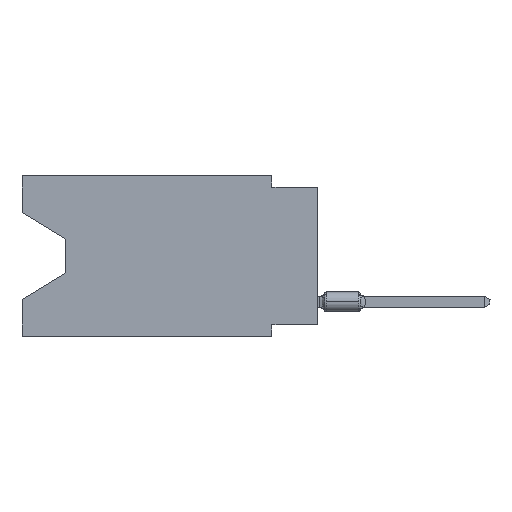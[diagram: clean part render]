
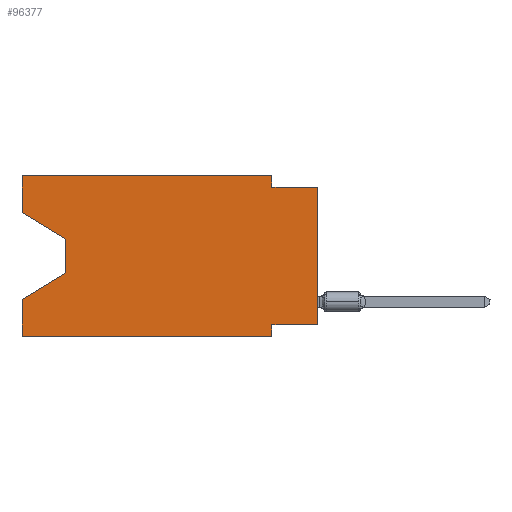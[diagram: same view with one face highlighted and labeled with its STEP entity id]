
A CAD part, left-side view. The second image highlights one B-rep face of the part: STEP entity #96377.
In plain terms, the highlighted planar face has unit normal (-1, 0, 0).
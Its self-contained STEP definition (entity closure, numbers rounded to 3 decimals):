
#4000 = EDGE_CURVE ( 'NONE', #24201, #12619, #29725, .T. ) ;
#5384 = LINE ( 'NONE', #61305, #67205 ) ;
#8667 = ORIENTED_EDGE ( 'NONE', *, *, #61540, .F. ) ;
#9030 = VERTEX_POINT ( 'NONE', #35441 ) ;
#9311 = CARTESIAN_POINT ( 'NONE',  ( 0., 2.54, 0. ) ) ;
#9453 = VECTOR ( 'NONE', #21239, 1000. ) ;
#11814 = AXIS2_PLACEMENT_3D ( 'NONE', #53244, #22499, #74934 ) ;
#12328 = CARTESIAN_POINT ( 'NONE',  ( 0., 16.383, -8.89 ) ) ;
#12422 = CARTESIAN_POINT ( 'NONE',  ( 0., 13.97, -3.505 ) ) ;
#12619 = VERTEX_POINT ( 'NONE', #95103 ) ;
#12642 = LINE ( 'NONE', #27778, #80653 ) ;
#12911 = DIRECTION ( 'NONE',  ( 0., 0., 1. ) ) ;
#13414 = CARTESIAN_POINT ( 'NONE',  ( 0., 0., 0. ) ) ;
#13535 = EDGE_CURVE ( 'NONE', #70506, #37479, #15150, .T. ) ;
#14707 = ORIENTED_EDGE ( 'NONE', *, *, #13535, .F. ) ;
#14742 = EDGE_CURVE ( 'NONE', #97646, #92942, #74917, .T. ) ;
#15150 = LINE ( 'NONE', #37864, #9453 ) ;
#18171 = VERTEX_POINT ( 'NONE', #9311 ) ;
#20701 = CARTESIAN_POINT ( 'NONE',  ( 0., 16.383, 0. ) ) ;
#20739 = DIRECTION ( 'NONE',  ( 0., -1., 0. ) ) ;
#20924 = VECTOR ( 'NONE', #30051, 1000. ) ;
#21239 = DIRECTION ( 'NONE',  ( 0., 0., -1. ) ) ;
#22499 = DIRECTION ( 'NONE',  ( 1., 0., 0. ) ) ;
#24201 = VERTEX_POINT ( 'NONE', #43690 ) ;
#24605 = CARTESIAN_POINT ( 'NONE',  ( 0., 16.383, -6.852 ) ) ;
#25156 = VERTEX_POINT ( 'NONE', #47427 ) ;
#25618 = VECTOR ( 'NONE', #96000, 1000. ) ;
#26809 = DIRECTION ( 'NONE',  ( 0., 0., -1. ) ) ;
#26849 = ORIENTED_EDGE ( 'NONE', *, *, #30157, .T. ) ;
#27102 = EDGE_CURVE ( 'NONE', #25156, #48154, #12642, .T. ) ;
#27778 = CARTESIAN_POINT ( 'NONE',  ( 0., 16.383, 0. ) ) ;
#28011 = CARTESIAN_POINT ( 'NONE',  ( 0., 13.97, -5.385 ) ) ;
#28906 = CARTESIAN_POINT ( 'NONE',  ( 0., 0., -8.255 ) ) ;
#29148 = ORIENTED_EDGE ( 'NONE', *, *, #45653, .F. ) ;
#29725 = LINE ( 'NONE', #76069, #42276 ) ;
#30051 = DIRECTION ( 'NONE',  ( 0., 0., 1. ) ) ;
#30157 = EDGE_CURVE ( 'NONE', #25156, #9030, #97678, .T. ) ;
#30634 = VECTOR ( 'NONE', #26809, 1000. ) ;
#32285 = LINE ( 'NONE', #12422, #36647 ) ;
#34878 = CARTESIAN_POINT ( 'NONE',  ( 0., 2.54, 0. ) ) ;
#35441 = CARTESIAN_POINT ( 'NONE',  ( 0., 13.97, -3.505 ) ) ;
#35876 = LINE ( 'NONE', #67103, #85628 ) ;
#36561 = ORIENTED_EDGE ( 'NONE', *, *, #84412, .T. ) ;
#36647 = VECTOR ( 'NONE', #65856, 1000. ) ;
#36966 = VECTOR ( 'NONE', #12911, 1000. ) ;
#37479 = VERTEX_POINT ( 'NONE', #87534 ) ;
#37864 = CARTESIAN_POINT ( 'NONE',  ( 0., 2.54, -8.89 ) ) ;
#39270 = DIRECTION ( 'NONE',  ( 0., -1., 0. ) ) ;
#40827 = CARTESIAN_POINT ( 'NONE',  ( 0., 2.54, -8.255 ) ) ;
#42276 = VECTOR ( 'NONE', #39270, 1000. ) ;
#43690 = CARTESIAN_POINT ( 'NONE',  ( 0., 2.54, -0.635 ) ) ;
#45653 = EDGE_CURVE ( 'NONE', #63135, #70506, #5384, .T. ) ;
#46171 = ORIENTED_EDGE ( 'NONE', *, *, #4000, .F. ) ;
#47427 = CARTESIAN_POINT ( 'NONE',  ( 0., 16.383, -2.038 ) ) ;
#48154 = VERTEX_POINT ( 'NONE', #84189 ) ;
#50703 = EDGE_CURVE ( 'NONE', #97646, #37479, #35876, .T. ) ;
#51859 = DIRECTION ( 'NONE',  ( 0., -0.855, -0.519 ) ) ;
#53244 = CARTESIAN_POINT ( 'NONE',  ( 0., 16.383, 0. ) ) ;
#53739 = FACE_OUTER_BOUND ( 'NONE', #76196, .T. ) ;
#57558 = ORIENTED_EDGE ( 'NONE', *, *, #90382, .T. ) ;
#59411 = CARTESIAN_POINT ( 'NONE',  ( 0., 16.383, -2.038 ) ) ;
#59505 = DIRECTION ( 'NONE',  ( 0., -1., 0. ) ) ;
#59524 = DIRECTION ( 'NONE',  ( 0., 0., 1. ) ) ;
#60547 = EDGE_CURVE ( 'NONE', #85233, #92942, #97007, .T. ) ;
#61305 = CARTESIAN_POINT ( 'NONE',  ( 0., 0., -8.255 ) ) ;
#61540 = EDGE_CURVE ( 'NONE', #48154, #18171, #89731, .T. ) ;
#61944 = ORIENTED_EDGE ( 'NONE', *, *, #91007, .F. ) ;
#63135 = VERTEX_POINT ( 'NONE', #28906 ) ;
#65856 = DIRECTION ( 'NONE',  ( 0., 0., -1. ) ) ;
#67103 = CARTESIAN_POINT ( 'NONE',  ( 0., 16.383, -8.89 ) ) ;
#67205 = VECTOR ( 'NONE', #76428, 1000. ) ;
#70506 = VERTEX_POINT ( 'NONE', #40827 ) ;
#73911 = CARTESIAN_POINT ( 'NONE',  ( 0., 16.383, 0. ) ) ;
#74917 = LINE ( 'NONE', #73911, #36966 ) ;
#74934 = DIRECTION ( 'NONE',  ( 0., 0., -1. ) ) ;
#76069 = CARTESIAN_POINT ( 'NONE',  ( 0., 0., -0.635 ) ) ;
#76196 = EDGE_LOOP ( 'NONE', ( #26849, #36561, #86576, #77764, #98702, #14707, #29148, #57558, #46171, #61944, #8667, #98672 ) ) ;
#76428 = DIRECTION ( 'NONE',  ( 0., 1., 0. ) ) ;
#77764 = ORIENTED_EDGE ( 'NONE', *, *, #14742, .F. ) ;
#79929 = VECTOR ( 'NONE', #51859, 1000. ) ;
#80653 = VECTOR ( 'NONE', #59524, 1000. ) ;
#82483 = PLANE ( 'NONE',  #11814 ) ;
#84189 = CARTESIAN_POINT ( 'NONE',  ( 0., 16.383, 0. ) ) ;
#84412 = EDGE_CURVE ( 'NONE', #9030, #85233, #32285, .T. ) ;
#85233 = VERTEX_POINT ( 'NONE', #96333 ) ;
#85628 = VECTOR ( 'NONE', #20739, 1000. ) ;
#86576 = ORIENTED_EDGE ( 'NONE', *, *, #60547, .T. ) ;
#87534 = CARTESIAN_POINT ( 'NONE',  ( 0., 2.54, -8.89 ) ) ;
#89731 = LINE ( 'NONE', #20701, #91658 ) ;
#90382 = EDGE_CURVE ( 'NONE', #63135, #12619, #99055, .T. ) ;
#91007 = EDGE_CURVE ( 'NONE', #18171, #24201, #95812, .T. ) ;
#91658 = VECTOR ( 'NONE', #59505, 1000. ) ;
#92942 = VERTEX_POINT ( 'NONE', #24605 ) ;
#95103 = CARTESIAN_POINT ( 'NONE',  ( 0., 0., -0.635 ) ) ;
#95812 = LINE ( 'NONE', #34878, #30634 ) ;
#96000 = DIRECTION ( 'NONE',  ( 0., 0.855, -0.519 ) ) ;
#96333 = CARTESIAN_POINT ( 'NONE',  ( 0., 13.97, -5.385 ) ) ;
#96377 = ADVANCED_FACE ( 'NONE', ( #53739 ), #82483, .F. ) ;
#97007 = LINE ( 'NONE', #28011, #25618 ) ;
#97646 = VERTEX_POINT ( 'NONE', #12328 ) ;
#97678 = LINE ( 'NONE', #59411, #79929 ) ;
#98672 = ORIENTED_EDGE ( 'NONE', *, *, #27102, .F. ) ;
#98702 = ORIENTED_EDGE ( 'NONE', *, *, #50703, .T. ) ;
#99055 = LINE ( 'NONE', #13414, #20924 ) ;
